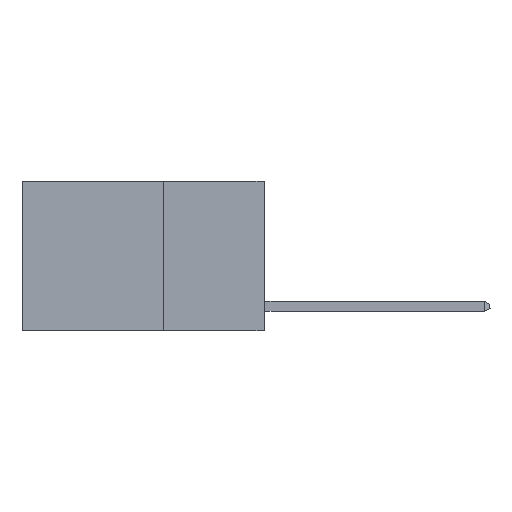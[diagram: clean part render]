
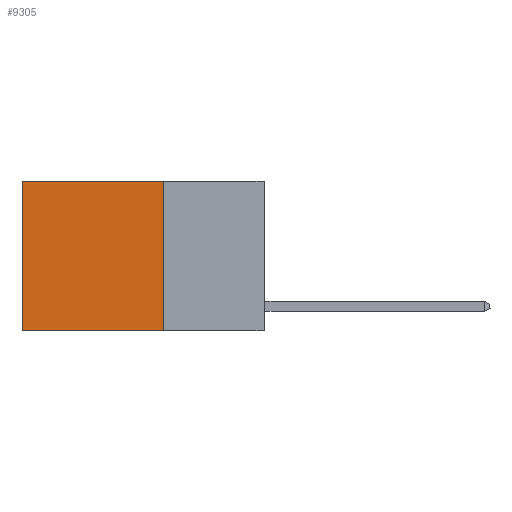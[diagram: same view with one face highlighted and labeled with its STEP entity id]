
A CAD part, left-side view. The second image highlights one B-rep face of the part: STEP entity #9305.
In plain terms, the highlighted planar face has unit normal (-1, 0, 0).
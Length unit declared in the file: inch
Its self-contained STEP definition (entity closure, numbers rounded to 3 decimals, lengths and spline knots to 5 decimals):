
#1469 = ORIENTED_EDGE ( 'NONE', *, *, #22012, .F. ) ;
#1817 = EDGE_CURVE ( 'NONE', #24328, #19175, #12831, .T. ) ;
#2949 = VECTOR ( 'NONE', #19112, 39.37008 ) ;
#2996 = CARTESIAN_POINT ( 'NONE',  ( 0.2625, 0.25, 0. ) ) ;
#3405 = CARTESIAN_POINT ( 'NONE',  ( 0.2625, 0.6, -0.37 ) ) ;
#3934 = VECTOR ( 'NONE', #6206, 39.37008 ) ;
#4399 = FACE_OUTER_BOUND ( 'NONE', #8487, .T. ) ;
#6206 = DIRECTION ( 'NONE',  ( 0., 0., -1. ) ) ;
#8487 = EDGE_LOOP ( 'NONE', ( #21681, #8772, #1469, #23228 ) ) ;
#8593 = VECTOR ( 'NONE', #22324, 39.37008 ) ;
#8772 = ORIENTED_EDGE ( 'NONE', *, *, #14774, .F. ) ;
#9305 = ADVANCED_FACE ( 'NONE', ( #4399 ), #9799, .F. ) ;
#9799 = PLANE ( 'NONE',  #11222 ) ;
#10041 = DIRECTION ( 'NONE',  ( 1., 0., 0. ) ) ;
#10596 = CARTESIAN_POINT ( 'NONE',  ( 0.2625, 0.25, -0.37 ) ) ;
#10819 = VERTEX_POINT ( 'NONE', #2996 ) ;
#11222 = AXIS2_PLACEMENT_3D ( 'NONE', #11540, #10041, #19102 ) ;
#11540 = CARTESIAN_POINT ( 'NONE',  ( 0.2625, 0.25, 0. ) ) ;
#11548 = CARTESIAN_POINT ( 'NONE',  ( 0.2625, 0.25, -0.37 ) ) ;
#12104 = CARTESIAN_POINT ( 'NONE',  ( 0.2625, 0.6, 0. ) ) ;
#12831 = LINE ( 'NONE', #20403, #18345 ) ;
#14750 = LINE ( 'NONE', #24299, #8593 ) ;
#14774 = EDGE_CURVE ( 'NONE', #21261, #19175, #24422, .T. ) ;
#17398 = CARTESIAN_POINT ( 'NONE',  ( 0.2625, 0.25, 0. ) ) ;
#18345 = VECTOR ( 'NONE', #23974, 39.37008 ) ;
#18711 = EDGE_CURVE ( 'NONE', #10819, #24328, #14750, .T. ) ;
#19102 = DIRECTION ( 'NONE',  ( 0., 0., -1. ) ) ;
#19112 = DIRECTION ( 'NONE',  ( 0., 1., 0. ) ) ;
#19175 = VERTEX_POINT ( 'NONE', #3405 ) ;
#20403 = CARTESIAN_POINT ( 'NONE',  ( 0.2625, 0.6, 0. ) ) ;
#21261 = VERTEX_POINT ( 'NONE', #10596 ) ;
#21681 = ORIENTED_EDGE ( 'NONE', *, *, #1817, .T. ) ;
#22012 = EDGE_CURVE ( 'NONE', #10819, #21261, #23220, .T. ) ;
#22324 = DIRECTION ( 'NONE',  ( 0., 1., 0. ) ) ;
#23220 = LINE ( 'NONE', #17398, #3934 ) ;
#23228 = ORIENTED_EDGE ( 'NONE', *, *, #18711, .T. ) ;
#23974 = DIRECTION ( 'NONE',  ( 0., 0., -1. ) ) ;
#24299 = CARTESIAN_POINT ( 'NONE',  ( 0.2625, 0.25, 0. ) ) ;
#24328 = VERTEX_POINT ( 'NONE', #12104 ) ;
#24422 = LINE ( 'NONE', #11548, #2949 ) ;
